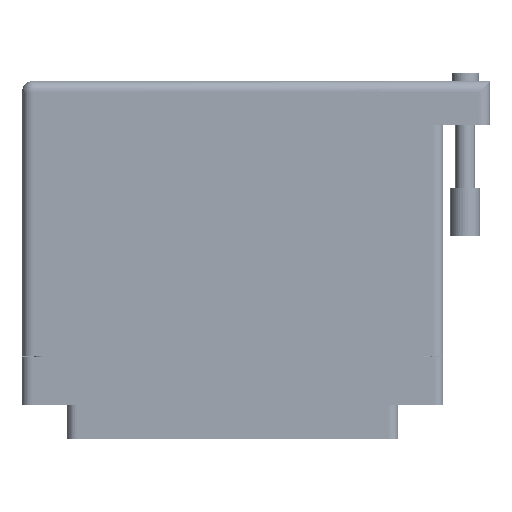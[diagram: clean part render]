
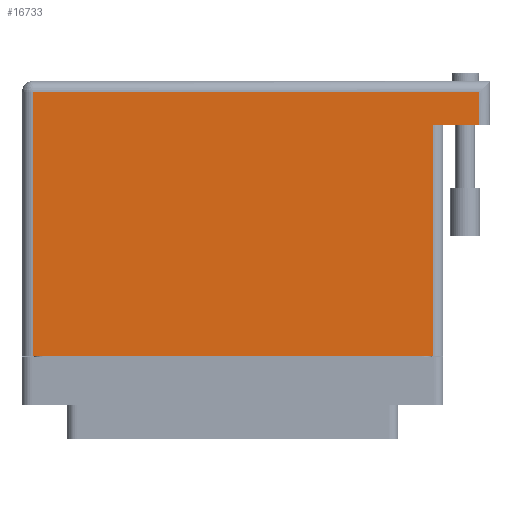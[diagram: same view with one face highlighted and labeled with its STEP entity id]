
A CAD part, front view. The second image highlights one B-rep face of the part: STEP entity #16733.
In plain terms, the highlighted face is planar.
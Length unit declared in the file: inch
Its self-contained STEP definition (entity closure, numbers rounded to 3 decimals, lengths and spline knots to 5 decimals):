
#5284 = EDGE_LOOP ( 'NONE', ( #10999, #31181, #22335, #6821, #43189, #48912 ) ) ;
#5918 = EDGE_CURVE ( 'NONE', #66864, #37776, #34293, .T. ) ;
#6821 = ORIENTED_EDGE ( 'NONE', *, *, #31422, .T. ) ;
#8328 = CARTESIAN_POINT ( 'NONE',  ( 1.289, 1.395, 0.617 ) ) ;
#10999 = ORIENTED_EDGE ( 'NONE', *, *, #47099, .T. ) ;
#15029 = CARTESIAN_POINT ( 'NONE',  ( 1.589, 1.605, 0.617 ) ) ;
#16733 = ADVANCED_FACE ( 'NONE', ( #40025 ), #71687, .F. ) ;
#17505 = LINE ( 'NONE', #18350, #33607 ) ;
#17922 = CARTESIAN_POINT ( 'NONE',  ( 1.289, 1.395, 0.617 ) ) ;
#18138 = AXIS2_PLACEMENT_3D ( 'NONE', #36923, #38868, #33119 ) ;
#18350 = CARTESIAN_POINT ( 'NONE',  ( -1.289, -0.1, 0.617 ) ) ;
#19125 = CARTESIAN_POINT ( 'NONE',  ( -1.289, -0.1, 0.617 ) ) ;
#19275 = VECTOR ( 'NONE', #41495, 39.37008 ) ;
#22335 = ORIENTED_EDGE ( 'NONE', *, *, #5918, .F. ) ;
#24664 = LINE ( 'NONE', #46909, #19275 ) ;
#27434 = CARTESIAN_POINT ( 'NONE',  ( -1.359, -0.1, 0.617 ) ) ;
#29679 = VERTEX_POINT ( 'NONE', #49128 ) ;
#30256 = DIRECTION ( 'NONE',  ( 0., -1., 0. ) ) ;
#30700 = VECTOR ( 'NONE', #33458, 39.37008 ) ;
#31181 = ORIENTED_EDGE ( 'NONE', *, *, #62454, .T. ) ;
#31422 = EDGE_CURVE ( 'NONE', #66864, #59839, #24664, .T. ) ;
#33119 = DIRECTION ( 'NONE',  ( -1., 0., 0. ) ) ;
#33458 = DIRECTION ( 'NONE',  ( -1., 0., 0. ) ) ;
#33607 = VECTOR ( 'NONE', #30256, 39.37008 ) ;
#34293 = LINE ( 'NONE', #61850, #30700 ) ;
#35040 = EDGE_CURVE ( 'NONE', #29679, #67445, #17505, .T. ) ;
#36923 = CARTESIAN_POINT ( 'NONE',  ( -1.359, 1.675, 0.617 ) ) ;
#37026 = LINE ( 'NONE', #27434, #63683 ) ;
#37776 = VERTEX_POINT ( 'NONE', #8328 ) ;
#38868 = DIRECTION ( 'NONE',  ( 0., 0., -1. ) ) ;
#40025 = FACE_OUTER_BOUND ( 'NONE', #5284, .T. ) ;
#41495 = DIRECTION ( 'NONE',  ( 0., 1., 0. ) ) ;
#43189 = ORIENTED_EDGE ( 'NONE', *, *, #53673, .T. ) ;
#46909 = CARTESIAN_POINT ( 'NONE',  ( 1.589, 1.675, 0.617 ) ) ;
#47099 = EDGE_CURVE ( 'NONE', #67445, #55993, #37026, .T. ) ;
#48912 = ORIENTED_EDGE ( 'NONE', *, *, #35040, .T. ) ;
#49128 = CARTESIAN_POINT ( 'NONE',  ( -1.289, 1.605, 0.617 ) ) ;
#50666 = VECTOR ( 'NONE', #57749, 39.37008 ) ;
#53673 = EDGE_CURVE ( 'NONE', #59839, #29679, #69898, .T. ) ;
#55993 = VERTEX_POINT ( 'NONE', #64621 ) ;
#57749 = DIRECTION ( 'NONE',  ( 0., 1., 0. ) ) ;
#59304 = CARTESIAN_POINT ( 'NONE',  ( -1.359, 1.605, 0.617 ) ) ;
#59839 = VERTEX_POINT ( 'NONE', #15029 ) ;
#61850 = CARTESIAN_POINT ( 'NONE',  ( 1.659, 1.395, 0.617 ) ) ;
#62454 = EDGE_CURVE ( 'NONE', #55993, #37776, #65839, .T. ) ;
#63683 = VECTOR ( 'NONE', #73234, 39.37008 ) ;
#64621 = CARTESIAN_POINT ( 'NONE',  ( 1.289, -0.1, 0.617 ) ) ;
#65275 = DIRECTION ( 'NONE',  ( -1., 0., 0. ) ) ;
#65524 = VECTOR ( 'NONE', #65275, 39.37008 ) ;
#65839 = LINE ( 'NONE', #17922, #50666 ) ;
#66864 = VERTEX_POINT ( 'NONE', #68055 ) ;
#67445 = VERTEX_POINT ( 'NONE', #19125 ) ;
#68055 = CARTESIAN_POINT ( 'NONE',  ( 1.589, 1.395, 0.617 ) ) ;
#69898 = LINE ( 'NONE', #59304, #65524 ) ;
#71687 = PLANE ( 'NONE',  #18138 ) ;
#73234 = DIRECTION ( 'NONE',  ( 1., 0., 0. ) ) ;
